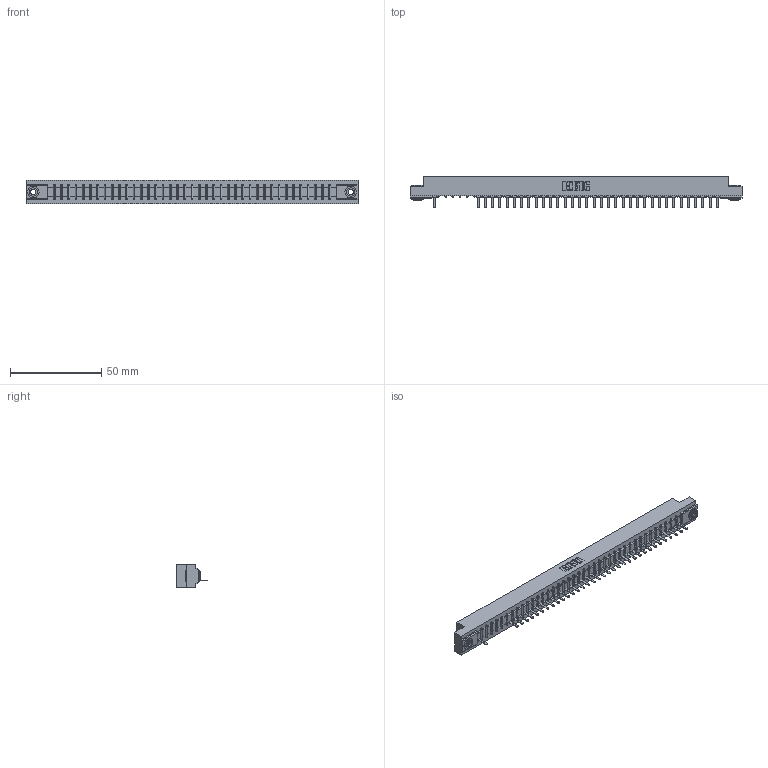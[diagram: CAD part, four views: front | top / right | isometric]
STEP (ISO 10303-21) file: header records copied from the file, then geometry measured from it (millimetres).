
FILE_DESCRIPTION (( 'STEP AP203' ), '1' );
FILE_NAME ('357-040-521-103.STEP', '2018-08-11T05:18:09', ( '' ), ( '' ), 'SwSTEP 2.0', 'SolidWorks 2016', '' );
FILE_SCHEMA (( 'CONFIG_CONTROL_DESIGN' ));
Length unit declared in the file: inch
Products named in the file (4): 307 Part_.156 Dia Mounting Holes; 307-290-002_521; 345-250-002_345-250-002-102; 357-040-521-103
Assembly tree (38 placements, depth 2):
  357-040-521-103
    307 Part_.156 Dia Mounting Holes
    307-290-002_521  x35
    345-250-002_345-250-002-102  x2
Bounding box: 181.51 x 17.42 x 12.7 mm (x, y, z)
Volume: 19267.4 mm3; surface area: 23510.6 mm2
Topology: 38 solids, 38 shells, 2901 faces, 8875 edges, 5802 vertices
Faces by surface type: plane 1729, cylinder 1082, sphere 82, cone 8
Entity records: 36161 total; most frequent: CARTESIAN_POINT 6100, ORIENTED_EDGE 6086, DIRECTION 5937, EDGE_CURVE 3043, VECTOR 2323, LINE 2323, VERTEX_POINT 1970, AXIS2_PLACEMENT_3D 1807
